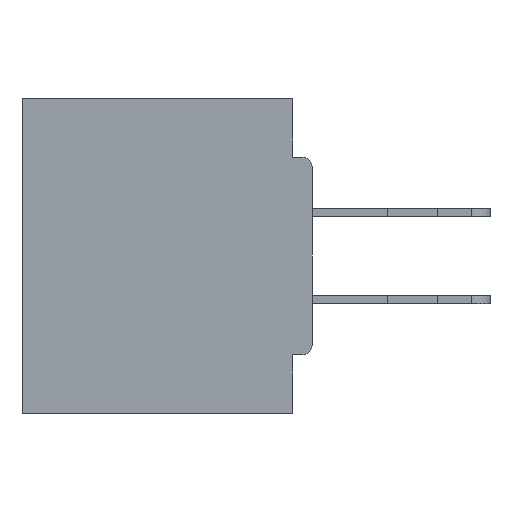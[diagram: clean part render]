
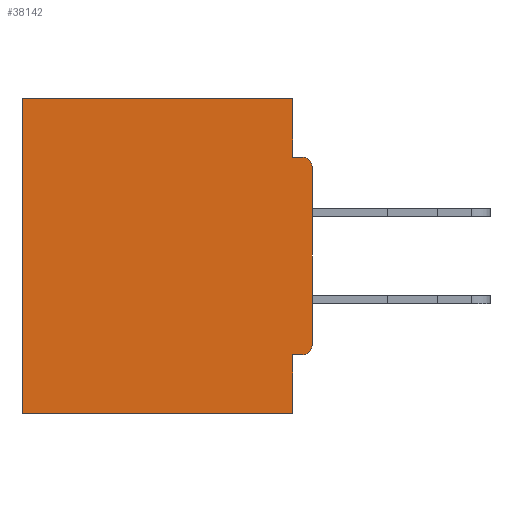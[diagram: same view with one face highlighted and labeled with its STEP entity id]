
A CAD part, left-side view. The second image highlights one B-rep face of the part: STEP entity #38142.
In plain terms, the highlighted planar face has unit normal (-1, 0, 0).
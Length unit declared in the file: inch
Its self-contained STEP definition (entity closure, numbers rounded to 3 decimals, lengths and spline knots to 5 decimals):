
#541 = LINE ( 'NONE', #38400, #11510 ) ;
#829 = DIRECTION ( 'NONE',  ( 0., 0., -1. ) ) ;
#2068 = CARTESIAN_POINT ( 'NONE',  ( 0.298, 0.015, -0.0935 ) ) ;
#2101 = LINE ( 'NONE', #2387, #15432 ) ;
#2139 = CARTESIAN_POINT ( 'NONE',  ( 0.298, 0.031, -0.5 ) ) ;
#2387 = CARTESIAN_POINT ( 'NONE',  ( 0.298, 0., -0.5 ) ) ;
#2693 = VECTOR ( 'NONE', #829, 39.37008 ) ;
#2895 = CIRCLE ( 'NONE', #10153, 0.015 ) ;
#3027 = DIRECTION ( 'NONE',  ( -1., 0., 0. ) ) ;
#3898 = VECTOR ( 'NONE', #13514, 39.37008 ) ;
#4612 = EDGE_CURVE ( 'NONE', #32793, #34095, #25282, .T. ) ;
#4828 = CARTESIAN_POINT ( 'NONE',  ( 0.298, 0., -0.1085 ) ) ;
#5731 = AXIS2_PLACEMENT_3D ( 'NONE', #30399, #12636, #21730 ) ;
#7473 = VERTEX_POINT ( 'NONE', #19825 ) ;
#7629 = VERTEX_POINT ( 'NONE', #2139 ) ;
#7987 = VERTEX_POINT ( 'NONE', #31832 ) ;
#9091 = EDGE_CURVE ( 'NONE', #7629, #7473, #2101, .T. ) ;
#9257 = ORIENTED_EDGE ( 'NONE', *, *, #4612, .F. ) ;
#9792 = ORIENTED_EDGE ( 'NONE', *, *, #34470, .F. ) ;
#10153 = AXIS2_PLACEMENT_3D ( 'NONE', #35772, #29406, #29786 ) ;
#10226 = CARTESIAN_POINT ( 'NONE',  ( 0.298, 0.46, 0. ) ) ;
#10323 = CARTESIAN_POINT ( 'NONE',  ( 0.298, 0.46, 0. ) ) ;
#11091 = EDGE_CURVE ( 'NONE', #23449, #34738, #17963, .T. ) ;
#11346 = VECTOR ( 'NONE', #23172, 39.37008 ) ;
#11368 = VECTOR ( 'NONE', #36825, 39.37008 ) ;
#11397 = EDGE_LOOP ( 'NONE', ( #13968, #9257, #16491, #21716, #38682, #24957, #9792, #25917, #36974, #32258 ) ) ;
#11510 = VECTOR ( 'NONE', #15095, 39.37008 ) ;
#12636 = DIRECTION ( 'NONE',  ( 1., 0., 0. ) ) ;
#13278 = LINE ( 'NONE', #24534, #11368 ) ;
#13514 = DIRECTION ( 'NONE',  ( 0., -1., 0. ) ) ;
#13517 = AXIS2_PLACEMENT_3D ( 'NONE', #21212, #3027, #21334 ) ;
#13968 = ORIENTED_EDGE ( 'NONE', *, *, #30984, .T. ) ;
#14572 = EDGE_CURVE ( 'NONE', #37135, #7473, #34277, .T. ) ;
#14716 = FACE_OUTER_BOUND ( 'NONE', #11397, .T. ) ;
#15095 = DIRECTION ( 'NONE',  ( 0., 1., 0. ) ) ;
#15432 = VECTOR ( 'NONE', #33340, 39.37008 ) ;
#15455 = EDGE_CURVE ( 'NONE', #7987, #34738, #2895, .T. ) ;
#15771 = VECTOR ( 'NONE', #37736, 39.37008 ) ;
#16491 = ORIENTED_EDGE ( 'NONE', *, *, #34829, .F. ) ;
#17373 = CARTESIAN_POINT ( 'NONE',  ( 0.298, 0., 0. ) ) ;
#17963 = LINE ( 'NONE', #17373, #11346 ) ;
#18128 = VERTEX_POINT ( 'NONE', #21313 ) ;
#18644 = DIRECTION ( 'NONE',  ( 0., 0., -1. ) ) ;
#19709 = CARTESIAN_POINT ( 'NONE',  ( 0.298, 0.031, -0.0935 ) ) ;
#19825 = CARTESIAN_POINT ( 'NONE',  ( 0.298, 0.46, -0.5 ) ) ;
#21212 = CARTESIAN_POINT ( 'NONE',  ( 0.298, 0.015, -0.1085 ) ) ;
#21313 = CARTESIAN_POINT ( 'NONE',  ( 0.298, 0.031, -0.4065 ) ) ;
#21334 = DIRECTION ( 'NONE',  ( 0., 0., -1. ) ) ;
#21716 = ORIENTED_EDGE ( 'NONE', *, *, #31396, .T. ) ;
#21730 = DIRECTION ( 'NONE',  ( 0., 0., -1. ) ) ;
#23172 = DIRECTION ( 'NONE',  ( 0., 0., -1. ) ) ;
#23369 = CARTESIAN_POINT ( 'NONE',  ( 0.298, 0., -0.3915 ) ) ;
#23449 = VERTEX_POINT ( 'NONE', #4828 ) ;
#24534 = CARTESIAN_POINT ( 'NONE',  ( 0.298, 0., -0.4065 ) ) ;
#24957 = ORIENTED_EDGE ( 'NONE', *, *, #9091, .F. ) ;
#25282 = LINE ( 'NONE', #28377, #3898 ) ;
#25917 = ORIENTED_EDGE ( 'NONE', *, *, #33663, .F. ) ;
#25977 = LINE ( 'NONE', #38870, #30243 ) ;
#28377 = CARTESIAN_POINT ( 'NONE',  ( 0.298, 0., -0.0935 ) ) ;
#28852 = LINE ( 'NONE', #34320, #2693 ) ;
#29406 = DIRECTION ( 'NONE',  ( -1., 0., 0. ) ) ;
#29786 = DIRECTION ( 'NONE',  ( 0., 0., -1. ) ) ;
#30243 = VECTOR ( 'NONE', #18644, 39.37008 ) ;
#30399 = CARTESIAN_POINT ( 'NONE',  ( 0.298, 0., 0. ) ) ;
#30984 = EDGE_CURVE ( 'NONE', #23449, #34095, #38201, .T. ) ;
#31396 = EDGE_CURVE ( 'NONE', #32638, #37135, #541, .T. ) ;
#31832 = CARTESIAN_POINT ( 'NONE',  ( 0.298, 0.015, -0.4065 ) ) ;
#32258 = ORIENTED_EDGE ( 'NONE', *, *, #11091, .F. ) ;
#32638 = VERTEX_POINT ( 'NONE', #33573 ) ;
#32793 = VERTEX_POINT ( 'NONE', #19709 ) ;
#33314 = PLANE ( 'NONE',  #5731 ) ;
#33340 = DIRECTION ( 'NONE',  ( 0., 1., 0. ) ) ;
#33573 = CARTESIAN_POINT ( 'NONE',  ( 0.298, 0.031, 0. ) ) ;
#33663 = EDGE_CURVE ( 'NONE', #7987, #18128, #13278, .T. ) ;
#34095 = VERTEX_POINT ( 'NONE', #2068 ) ;
#34277 = LINE ( 'NONE', #10323, #15771 ) ;
#34320 = CARTESIAN_POINT ( 'NONE',  ( 0.298, 0.031, -0.5 ) ) ;
#34470 = EDGE_CURVE ( 'NONE', #18128, #7629, #28852, .T. ) ;
#34738 = VERTEX_POINT ( 'NONE', #23369 ) ;
#34829 = EDGE_CURVE ( 'NONE', #32638, #32793, #25977, .T. ) ;
#35772 = CARTESIAN_POINT ( 'NONE',  ( 0.298, 0.015, -0.3915 ) ) ;
#36825 = DIRECTION ( 'NONE',  ( 0., 1., 0. ) ) ;
#36974 = ORIENTED_EDGE ( 'NONE', *, *, #15455, .T. ) ;
#37135 = VERTEX_POINT ( 'NONE', #10226 ) ;
#37736 = DIRECTION ( 'NONE',  ( 0., 0., -1. ) ) ;
#38142 = ADVANCED_FACE ( 'NONE', ( #14716 ), #33314, .F. ) ;
#38201 = CIRCLE ( 'NONE', #13517, 0.015 ) ;
#38400 = CARTESIAN_POINT ( 'NONE',  ( 0.298, 0., 0. ) ) ;
#38682 = ORIENTED_EDGE ( 'NONE', *, *, #14572, .T. ) ;
#38870 = CARTESIAN_POINT ( 'NONE',  ( 0.298, 0.031, -0.5 ) ) ;
